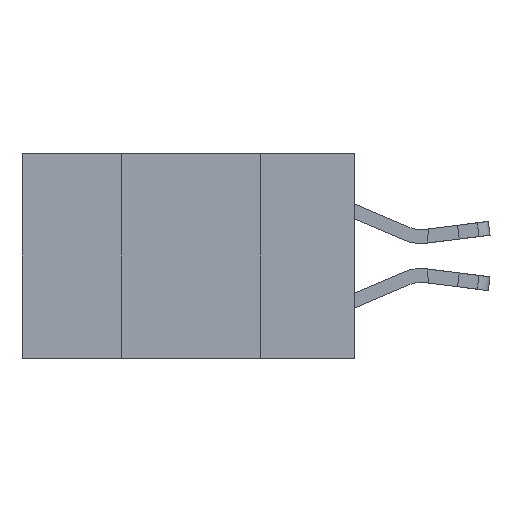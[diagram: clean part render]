
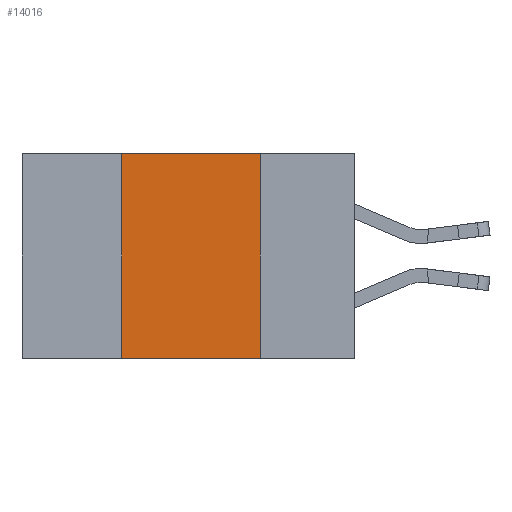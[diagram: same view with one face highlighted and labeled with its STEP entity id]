
A CAD part, left-side view. The second image highlights one B-rep face of the part: STEP entity #14016.
In plain terms, the highlighted planar face has unit normal (-1, 0, 0).
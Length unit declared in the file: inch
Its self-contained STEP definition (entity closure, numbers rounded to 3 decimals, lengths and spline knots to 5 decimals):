
#911 = ORIENTED_EDGE ( 'NONE', *, *, #25491, .T. ) ;
#2192 = CARTESIAN_POINT ( 'NONE',  ( 0., 0.17, -0.37 ) ) ;
#2231 = VERTEX_POINT ( 'NONE', #21072 ) ;
#3127 = CARTESIAN_POINT ( 'NONE',  ( 0., 0.17, 0. ) ) ;
#3616 = VECTOR ( 'NONE', #26246, 39.37008 ) ;
#4419 = LINE ( 'NONE', #21164, #20250 ) ;
#6029 = CARTESIAN_POINT ( 'NONE',  ( 0., 0.42, -0.37 ) ) ;
#7559 = EDGE_CURVE ( 'NONE', #23991, #12503, #4419, .T. ) ;
#8748 = DIRECTION ( 'NONE',  ( 0., 0., 1. ) ) ;
#9059 = DIRECTION ( 'NONE',  ( 1., 0., 0. ) ) ;
#10658 = DIRECTION ( 'NONE',  ( 0., 0., -1. ) ) ;
#12503 = VERTEX_POINT ( 'NONE', #2192 ) ;
#13558 = VECTOR ( 'NONE', #8748, 39.37008 ) ;
#14016 = ADVANCED_FACE ( 'NONE', ( #26614 ), #15276, .F. ) ;
#15276 = PLANE ( 'NONE',  #16161 ) ;
#15606 = EDGE_CURVE ( 'NONE', #2231, #23991, #20425, .T. ) ;
#16161 = AXIS2_PLACEMENT_3D ( 'NONE', #21658, #9059, #23764 ) ;
#18079 = EDGE_LOOP ( 'NONE', ( #21159, #22406, #21369, #911 ) ) ;
#19337 = EDGE_CURVE ( 'NONE', #25617, #2231, #19858, .T. ) ;
#19858 = LINE ( 'NONE', #25547, #13558 ) ;
#20250 = VECTOR ( 'NONE', #10658, 39.37008 ) ;
#20425 = LINE ( 'NONE', #24149, #3616 ) ;
#21072 = CARTESIAN_POINT ( 'NONE',  ( 0., 0.42, 0. ) ) ;
#21159 = ORIENTED_EDGE ( 'NONE', *, *, #7559, .F. ) ;
#21164 = CARTESIAN_POINT ( 'NONE',  ( 0., 0.17, 0. ) ) ;
#21369 = ORIENTED_EDGE ( 'NONE', *, *, #19337, .F. ) ;
#21658 = CARTESIAN_POINT ( 'NONE',  ( 0., 0.6, 0. ) ) ;
#22406 = ORIENTED_EDGE ( 'NONE', *, *, #15606, .F. ) ;
#22471 = DIRECTION ( 'NONE',  ( 0., -1., 0. ) ) ;
#23764 = DIRECTION ( 'NONE',  ( 0., 0., -1. ) ) ;
#23991 = VERTEX_POINT ( 'NONE', #3127 ) ;
#24149 = CARTESIAN_POINT ( 'NONE',  ( 0., 0.6, 0. ) ) ;
#24565 = CARTESIAN_POINT ( 'NONE',  ( 0., 0.6, -0.37 ) ) ;
#24716 = VECTOR ( 'NONE', #22471, 39.37008 ) ;
#25388 = LINE ( 'NONE', #24565, #24716 ) ;
#25491 = EDGE_CURVE ( 'NONE', #25617, #12503, #25388, .T. ) ;
#25547 = CARTESIAN_POINT ( 'NONE',  ( 0., 0.42, 0. ) ) ;
#25617 = VERTEX_POINT ( 'NONE', #6029 ) ;
#26246 = DIRECTION ( 'NONE',  ( 0., -1., 0. ) ) ;
#26614 = FACE_OUTER_BOUND ( 'NONE', #18079, .T. ) ;
